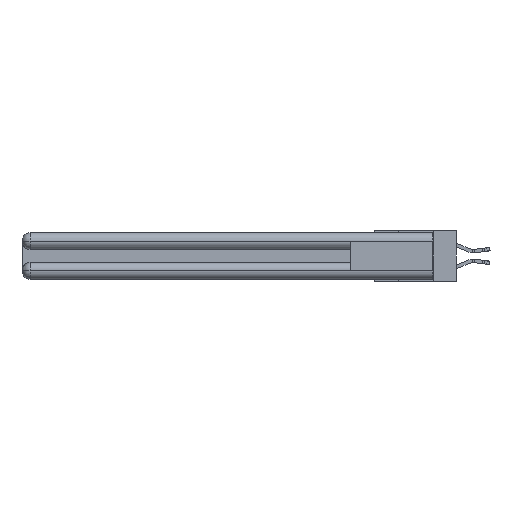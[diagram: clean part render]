
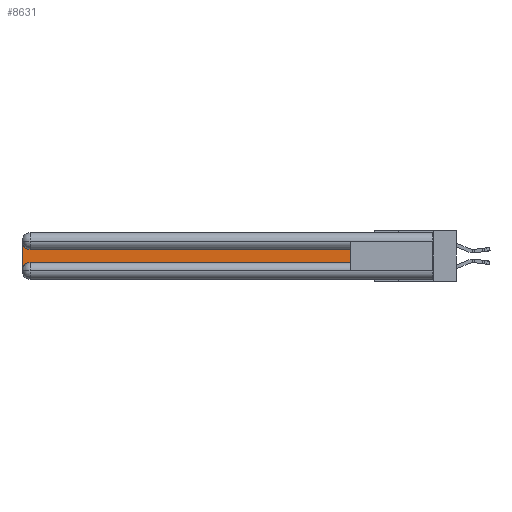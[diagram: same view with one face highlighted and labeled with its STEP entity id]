
A CAD part, left-side view. The second image highlights one B-rep face of the part: STEP entity #8631.
In plain terms, the highlighted planar face has unit normal (-1, 0, 0).
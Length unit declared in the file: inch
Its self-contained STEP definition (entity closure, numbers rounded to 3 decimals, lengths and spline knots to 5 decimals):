
#900 = EDGE_LOOP ( 'NONE', ( #22179, #23761, #21090, #18096, #10469, #12228 ) ) ;
#1000 = AXIS2_PLACEMENT_3D ( 'NONE', #15394, #2521, #10522 ) ;
#2449 = VERTEX_POINT ( 'NONE', #2999 ) ;
#2521 = DIRECTION ( 'NONE',  ( 1., 0., 0. ) ) ;
#2999 = CARTESIAN_POINT ( 'NONE',  ( 0.075, 0.6, -0.1225 ) ) ;
#3336 = CIRCLE ( 'NONE', #1000, 0.06 ) ;
#4262 = EDGE_CURVE ( 'NONE', #2449, #26231, #9361, .T. ) ;
#4671 = LINE ( 'NONE', #26216, #17915 ) ;
#5095 = DIRECTION ( 'NONE',  ( 0., 0., -1. ) ) ;
#6265 = CARTESIAN_POINT ( 'NONE',  ( 0.075, 3., -0.2775 ) ) ;
#6550 = AXIS2_PLACEMENT_3D ( 'NONE', #6849, #33557, #14968 ) ;
#6629 = VERTEX_POINT ( 'NONE', #15102 ) ;
#6849 = CARTESIAN_POINT ( 'NONE',  ( 0.075, 2.94, -0.2775 ) ) ;
#8614 = EDGE_CURVE ( 'NONE', #6629, #25345, #4671, .T. ) ;
#8631 = ADVANCED_FACE ( 'NONE', ( #28726 ), #29104, .F. ) ;
#8729 = CARTESIAN_POINT ( 'NONE',  ( 0.075, 0.6, -0.2175 ) ) ;
#9015 = LINE ( 'NONE', #10752, #21084 ) ;
#9361 = LINE ( 'NONE', #24821, #13930 ) ;
#10036 = EDGE_CURVE ( 'NONE', #26231, #14829, #3336, .T. ) ;
#10289 = CARTESIAN_POINT ( 'NONE',  ( 0.075, 3., -0.1225 ) ) ;
#10469 = ORIENTED_EDGE ( 'NONE', *, *, #8614, .T. ) ;
#10522 = DIRECTION ( 'NONE',  ( 0., 0., -1. ) ) ;
#10752 = CARTESIAN_POINT ( 'NONE',  ( 0.075, 3., -0.2175 ) ) ;
#11088 = DIRECTION ( 'NONE',  ( 0., 0., -1. ) ) ;
#11213 = EDGE_CURVE ( 'NONE', #12157, #6629, #34030, .T. ) ;
#11375 = EDGE_CURVE ( 'NONE', #25345, #2449, #13646, .T. ) ;
#12157 = VERTEX_POINT ( 'NONE', #6265 ) ;
#12228 = ORIENTED_EDGE ( 'NONE', *, *, #11375, .T. ) ;
#13005 = DIRECTION ( 'NONE',  ( 1., 0., 0. ) ) ;
#13646 = LINE ( 'NONE', #28655, #21915 ) ;
#13930 = VECTOR ( 'NONE', #19738, 39.37008 ) ;
#14829 = VERTEX_POINT ( 'NONE', #27034 ) ;
#14968 = DIRECTION ( 'NONE',  ( 0., 0., -1. ) ) ;
#15102 = CARTESIAN_POINT ( 'NONE',  ( 0.075, 2.94, -0.2175 ) ) ;
#15196 = DIRECTION ( 'NONE',  ( 0., 0., 1. ) ) ;
#15394 = CARTESIAN_POINT ( 'NONE',  ( 0.075, 2.94, -0.0625 ) ) ;
#15985 = DIRECTION ( 'NONE',  ( 0., -1., 0. ) ) ;
#16908 = AXIS2_PLACEMENT_3D ( 'NONE', #10289, #13005, #5095 ) ;
#17915 = VECTOR ( 'NONE', #15985, 39.37008 ) ;
#18096 = ORIENTED_EDGE ( 'NONE', *, *, #11213, .T. ) ;
#19738 = DIRECTION ( 'NONE',  ( 0., 1., 0. ) ) ;
#21084 = VECTOR ( 'NONE', #11088, 39.37008 ) ;
#21090 = ORIENTED_EDGE ( 'NONE', *, *, #26931, .T. ) ;
#21915 = VECTOR ( 'NONE', #15196, 39.37008 ) ;
#22179 = ORIENTED_EDGE ( 'NONE', *, *, #4262, .T. ) ;
#23761 = ORIENTED_EDGE ( 'NONE', *, *, #10036, .T. ) ;
#24821 = CARTESIAN_POINT ( 'NONE',  ( 0.075, 0.6, -0.1225 ) ) ;
#25345 = VERTEX_POINT ( 'NONE', #8729 ) ;
#26216 = CARTESIAN_POINT ( 'NONE',  ( 0.075, 0.6, -0.2175 ) ) ;
#26231 = VERTEX_POINT ( 'NONE', #27577 ) ;
#26931 = EDGE_CURVE ( 'NONE', #14829, #12157, #9015, .T. ) ;
#27034 = CARTESIAN_POINT ( 'NONE',  ( 0.075, 3., -0.0625 ) ) ;
#27577 = CARTESIAN_POINT ( 'NONE',  ( 0.075, 2.94, -0.1225 ) ) ;
#28655 = CARTESIAN_POINT ( 'NONE',  ( 0.075, 0.6, -0.2175 ) ) ;
#28726 = FACE_OUTER_BOUND ( 'NONE', #900, .T. ) ;
#29104 = PLANE ( 'NONE',  #16908 ) ;
#33557 = DIRECTION ( 'NONE',  ( 1., 0., 0. ) ) ;
#34030 = CIRCLE ( 'NONE', #6550, 0.06 ) ;
